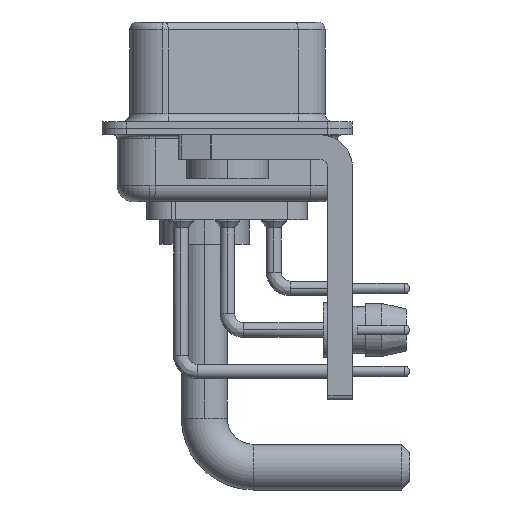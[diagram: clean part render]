
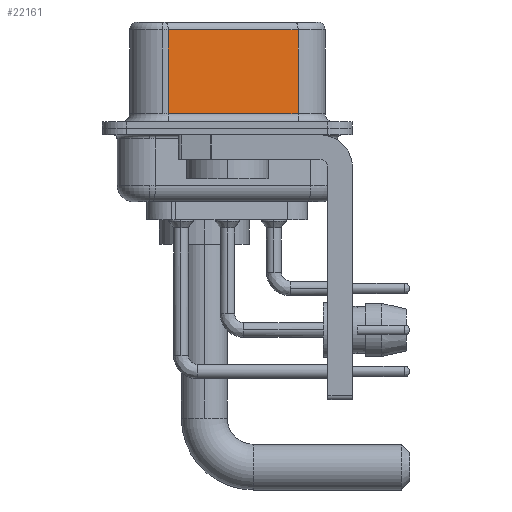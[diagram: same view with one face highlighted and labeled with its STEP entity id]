
A CAD part, left-side view. The second image highlights one B-rep face of the part: STEP entity #22161.
In plain terms, the highlighted planar face has unit normal (-0.985, -0.174, 0).
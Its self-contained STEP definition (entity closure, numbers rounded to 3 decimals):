
#1448 = DIRECTION ( 'NONE',  ( 0.985, 0.174, 0. ) ) ;
#3050 = CARTESIAN_POINT ( 'NONE',  ( 5.132, -4.322, 6.52 ) ) ;
#3207 = EDGE_CURVE ( 'NONE', #34172, #24999, #36999, .T. ) ;
#4104 = EDGE_CURVE ( 'NONE', #35716, #13060, #24372, .T. ) ;
#4294 = FACE_OUTER_BOUND ( 'NONE', #6310, .T. ) ;
#6310 = EDGE_LOOP ( 'NONE', ( #14917, #24878, #10956, #8562 ) ) ;
#8562 = ORIENTED_EDGE ( 'NONE', *, *, #27316, .T. ) ;
#9318 = DIRECTION ( 'NONE',  ( 0., 0., -1. ) ) ;
#10565 = CARTESIAN_POINT ( 'NONE',  ( 5.132, -4.322, 6.52 ) ) ;
#10766 = DIRECTION ( 'NONE',  ( -0.174, 0.985, 0. ) ) ;
#10956 = ORIENTED_EDGE ( 'NONE', *, *, #4104, .T. ) ;
#12476 = EDGE_CURVE ( 'NONE', #34172, #35716, #12689, .T. ) ;
#12689 = LINE ( 'NONE', #21772, #16877 ) ;
#13060 = VERTEX_POINT ( 'NONE', #37832 ) ;
#13798 = VECTOR ( 'NONE', #9318, 1000. ) ;
#14917 = ORIENTED_EDGE ( 'NONE', *, *, #3207, .F. ) ;
#15076 = CARTESIAN_POINT ( 'NONE',  ( 5.132, -4.322, 0.9 ) ) ;
#16877 = VECTOR ( 'NONE', #34094, 1000. ) ;
#17023 = VECTOR ( 'NONE', #18495, 1000. ) ;
#17592 = CARTESIAN_POINT ( 'NONE',  ( 3.73, 3.628, 6.02 ) ) ;
#18315 = DIRECTION ( 'NONE',  ( 0., 0., -1. ) ) ;
#18495 = DIRECTION ( 'NONE',  ( 0.174, -0.985, 0. ) ) ;
#19372 = CARTESIAN_POINT ( 'NONE',  ( 5.132, -4.322, 6.02 ) ) ;
#19443 = AXIS2_PLACEMENT_3D ( 'NONE', #10565, #1448, #10766 ) ;
#21772 = CARTESIAN_POINT ( 'NONE',  ( 5.132, -4.322, 6.02 ) ) ;
#22161 = ADVANCED_FACE ( 'NONE', ( #4294 ), #38038, .F. ) ;
#24351 = LINE ( 'NONE', #15076, #17023 ) ;
#24372 = LINE ( 'NONE', #33666, #32544 ) ;
#24878 = ORIENTED_EDGE ( 'NONE', *, *, #12476, .T. ) ;
#24999 = VERTEX_POINT ( 'NONE', #39488 ) ;
#27316 = EDGE_CURVE ( 'NONE', #13060, #24999, #24351, .T. ) ;
#32544 = VECTOR ( 'NONE', #18315, 1000. ) ;
#33666 = CARTESIAN_POINT ( 'NONE',  ( 3.73, 3.628, 6.52 ) ) ;
#34094 = DIRECTION ( 'NONE',  ( -0.174, 0.985, 0. ) ) ;
#34172 = VERTEX_POINT ( 'NONE', #19372 ) ;
#35716 = VERTEX_POINT ( 'NONE', #17592 ) ;
#36999 = LINE ( 'NONE', #3050, #13798 ) ;
#37832 = CARTESIAN_POINT ( 'NONE',  ( 3.73, 3.628, 0.9 ) ) ;
#38038 = PLANE ( 'NONE',  #19443 ) ;
#39488 = CARTESIAN_POINT ( 'NONE',  ( 5.132, -4.322, 0.9 ) ) ;
